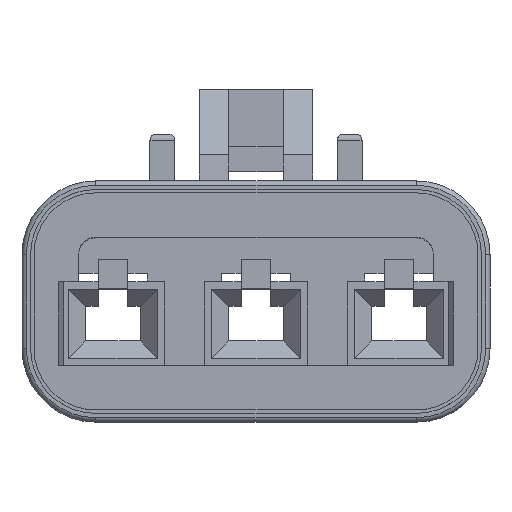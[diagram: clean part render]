
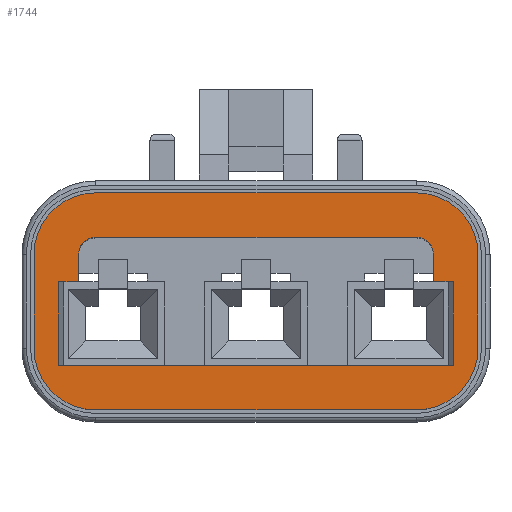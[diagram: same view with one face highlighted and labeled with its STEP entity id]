
A CAD part, top view. The second image highlights one B-rep face of the part: STEP entity #1744.
In plain terms, the highlighted planar face has unit normal (0, 0, 1).
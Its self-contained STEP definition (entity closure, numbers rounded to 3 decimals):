
#148 = VECTOR ( 'NONE', #1796, 1000. ) ;
#175 = AXIS2_PLACEMENT_3D ( 'NONE', #8669, #4275, #6469 ) ;
#259 = VECTOR ( 'NONE', #5581, 1000. ) ;
#351 = LINE ( 'NONE', #9261, #5116 ) ;
#423 = DIRECTION ( 'NONE',  ( 1., 0., 0. ) ) ;
#487 = EDGE_CURVE ( 'NONE', #14204, #9851, #10210, .T. ) ;
#541 = LINE ( 'NONE', #13019, #6979 ) ;
#652 = CARTESIAN_POINT ( 'NONE',  ( 7.2, 2.5, 26. ) ) ;
#702 = VERTEX_POINT ( 'NONE', #5740 ) ;
#755 = CARTESIAN_POINT ( 'NONE',  ( 9., 2.5, 26. ) ) ;
#783 = LINE ( 'NONE', #6271, #148 ) ;
#839 = FACE_BOUND ( 'NONE', #12326, .T. ) ;
#920 = CIRCLE ( 'NONE', #8642, 2.5 ) ;
#995 = DIRECTION ( 'NONE',  ( 0., 0., 1. ) ) ;
#1138 = AXIS2_PLACEMENT_3D ( 'NONE', #12852, #7104, #5040 ) ;
#1155 = ORIENTED_EDGE ( 'NONE', *, *, #10953, .F. ) ;
#1247 = ORIENTED_EDGE ( 'NONE', *, *, #12876, .T. ) ;
#1343 = ORIENTED_EDGE ( 'NONE', *, *, #2974, .T. ) ;
#1395 = DIRECTION ( 'NONE',  ( 0., 1., 0. ) ) ;
#1744 = ADVANCED_FACE ( 'NONE', ( #839, #4198 ), #1860, .T. ) ;
#1796 = DIRECTION ( 'NONE',  ( 1., 0., 0. ) ) ;
#1860 = PLANE ( 'NONE',  #175 ) ;
#2545 = CARTESIAN_POINT ( 'NONE',  ( 8., -2., 26. ) ) ;
#2555 = VECTOR ( 'NONE', #7586, 1000. ) ;
#2592 = LINE ( 'NONE', #5595, #9857 ) ;
#2964 = LINE ( 'NONE', #11877, #12336 ) ;
#2974 = EDGE_CURVE ( 'NONE', #7461, #9075, #12168, .T. ) ;
#3086 = CARTESIAN_POINT ( 'NONE',  ( -9., 2.5, 26. ) ) ;
#3341 = EDGE_CURVE ( 'NONE', #9075, #12950, #11338, .T. ) ;
#3458 = VERTEX_POINT ( 'NONE', #9221 ) ;
#3772 = VECTOR ( 'NONE', #4837, 1000. ) ;
#3777 = DIRECTION ( 'NONE',  ( 0., 0., 1. ) ) ;
#3880 = ORIENTED_EDGE ( 'NONE', *, *, #10201, .T. ) ;
#4079 = CARTESIAN_POINT ( 'NONE',  ( -6.5, 2.5, 26. ) ) ;
#4198 = FACE_OUTER_BOUND ( 'NONE', #9828, .T. ) ;
#4275 = DIRECTION ( 'NONE',  ( 0., 0., 1. ) ) ;
#4295 = ORIENTED_EDGE ( 'NONE', *, *, #10071, .F. ) ;
#4398 = ORIENTED_EDGE ( 'NONE', *, *, #11031, .T. ) ;
#4552 = VERTEX_POINT ( 'NONE', #5878 ) ;
#4837 = DIRECTION ( 'NONE',  ( -1., 0., 0. ) ) ;
#4908 = VERTEX_POINT ( 'NONE', #8935 ) ;
#4914 = DIRECTION ( 'NONE',  ( 0., 1., 0. ) ) ;
#4923 = VERTEX_POINT ( 'NONE', #6957 ) ;
#4965 = CARTESIAN_POINT ( 'NONE',  ( 9., -1.3, 26. ) ) ;
#5040 = DIRECTION ( 'NONE',  ( 1., 0., 0. ) ) ;
#5116 = VECTOR ( 'NONE', #423, 1000. ) ;
#5126 = VERTEX_POINT ( 'NONE', #7763 ) ;
#5185 = VERTEX_POINT ( 'NONE', #2545 ) ;
#5456 = DIRECTION ( 'NONE',  ( -1., 0., 0. ) ) ;
#5581 = DIRECTION ( 'NONE',  ( 0., -1., 0. ) ) ;
#5595 = CARTESIAN_POINT ( 'NONE',  ( 6.5, 5., 26. ) ) ;
#5720 = CARTESIAN_POINT ( 'NONE',  ( -9., 2.5, 26. ) ) ;
#5721 = CARTESIAN_POINT ( 'NONE',  ( 7.2, 1.4, 26. ) ) ;
#5740 = CARTESIAN_POINT ( 'NONE',  ( 6.5, -3.8, 26. ) ) ;
#5805 = VECTOR ( 'NONE', #4914, 1000. ) ;
#5843 = LINE ( 'NONE', #12065, #7610 ) ;
#5878 = CARTESIAN_POINT ( 'NONE',  ( -8., -2., 26. ) ) ;
#5934 = CARTESIAN_POINT ( 'NONE',  ( 6.5, 2.5, 26. ) ) ;
#6152 = ORIENTED_EDGE ( 'NONE', *, *, #9581, .F. ) ;
#6271 = CARTESIAN_POINT ( 'NONE',  ( 6.5, -3.8, 26. ) ) ;
#6279 = VERTEX_POINT ( 'NONE', #8212 ) ;
#6295 = ORIENTED_EDGE ( 'NONE', *, *, #7516, .T. ) ;
#6426 = DIRECTION ( 'NONE',  ( 1., 0., 0. ) ) ;
#6438 = CARTESIAN_POINT ( 'NONE',  ( 6.5, 2.5, 26. ) ) ;
#6469 = DIRECTION ( 'NONE',  ( 1., 0., 0. ) ) ;
#6522 = CIRCLE ( 'NONE', #1138, 2.5 ) ;
#6643 = AXIS2_PLACEMENT_3D ( 'NONE', #6438, #9850, #10873 ) ;
#6698 = DIRECTION ( 'NONE',  ( -1., 0., 0. ) ) ;
#6835 = ORIENTED_EDGE ( 'NONE', *, *, #14141, .T. ) ;
#6957 = CARTESIAN_POINT ( 'NONE',  ( -7.2, 1.4, 26. ) ) ;
#6965 = ORIENTED_EDGE ( 'NONE', *, *, #8897, .F. ) ;
#6979 = VECTOR ( 'NONE', #9442, 1000. ) ;
#7104 = DIRECTION ( 'NONE',  ( 0., 0., 1. ) ) ;
#7365 = CARTESIAN_POINT ( 'NONE',  ( -9., -1.3, 26. ) ) ;
#7435 = ORIENTED_EDGE ( 'NONE', *, *, #10886, .F. ) ;
#7461 = VERTEX_POINT ( 'NONE', #11205 ) ;
#7516 = EDGE_CURVE ( 'NONE', #6279, #7461, #2592, .T. ) ;
#7586 = DIRECTION ( 'NONE',  ( -1., 0., 0. ) ) ;
#7610 = VECTOR ( 'NONE', #14406, 1000. ) ;
#7743 = AXIS2_PLACEMENT_3D ( 'NONE', #10997, #995, #5456 ) ;
#7763 = CARTESIAN_POINT ( 'NONE',  ( 7.2, 1.4, 26. ) ) ;
#7981 = VERTEX_POINT ( 'NONE', #652 ) ;
#8002 = DIRECTION ( 'NONE',  ( 0., -1., 0. ) ) ;
#8136 = LINE ( 'NONE', #5721, #3772 ) ;
#8160 = CARTESIAN_POINT ( 'NONE',  ( 6.5, -1.3, 26. ) ) ;
#8212 = CARTESIAN_POINT ( 'NONE',  ( 6.5, 5., 26. ) ) ;
#8324 = DIRECTION ( 'NONE',  ( 0., 0., 1. ) ) ;
#8443 = EDGE_CURVE ( 'NONE', #5126, #7981, #13817, .T. ) ;
#8575 = LINE ( 'NONE', #755, #5805 ) ;
#8642 = AXIS2_PLACEMENT_3D ( 'NONE', #5934, #8951, #6698 ) ;
#8669 = CARTESIAN_POINT ( 'NONE',  ( -6.5, -1.3, 26. ) ) ;
#8880 = CARTESIAN_POINT ( 'NONE',  ( 9., 2.5, 26. ) ) ;
#8897 = EDGE_CURVE ( 'NONE', #4908, #5126, #8136, .T. ) ;
#8929 = ORIENTED_EDGE ( 'NONE', *, *, #3341, .T. ) ;
#8935 = CARTESIAN_POINT ( 'NONE',  ( 8., 1.4, 26. ) ) ;
#8951 = DIRECTION ( 'NONE',  ( 0., 0., 1. ) ) ;
#9015 = ORIENTED_EDGE ( 'NONE', *, *, #8443, .F. ) ;
#9028 = VERTEX_POINT ( 'NONE', #9574 ) ;
#9075 = VERTEX_POINT ( 'NONE', #3086 ) ;
#9085 = CARTESIAN_POINT ( 'NONE',  ( -7.2, 2.5, 26. ) ) ;
#9087 = ORIENTED_EDGE ( 'NONE', *, *, #487, .F. ) ;
#9192 = CIRCLE ( 'NONE', #6643, 0.7 ) ;
#9221 = CARTESIAN_POINT ( 'NONE',  ( 6.5, 3.2, 26. ) ) ;
#9261 = CARTESIAN_POINT ( 'NONE',  ( -6.5, -2., 26. ) ) ;
#9431 = VERTEX_POINT ( 'NONE', #4965 ) ;
#9442 = DIRECTION ( 'NONE',  ( 0., 1., 0. ) ) ;
#9484 = ORIENTED_EDGE ( 'NONE', *, *, #10559, .T. ) ;
#9574 = CARTESIAN_POINT ( 'NONE',  ( -8., 1.4, 26. ) ) ;
#9581 = EDGE_CURVE ( 'NONE', #7981, #3458, #9192, .T. ) ;
#9828 = EDGE_LOOP ( 'NONE', ( #9484, #6835, #1247, #3880, #4398, #6295, #1343, #8929 ) ) ;
#9850 = DIRECTION ( 'NONE',  ( 0., 0., 1. ) ) ;
#9851 = VERTEX_POINT ( 'NONE', #12078 ) ;
#9857 = VECTOR ( 'NONE', #12302, 1000. ) ;
#9895 = VERTEX_POINT ( 'NONE', #8880 ) ;
#10071 = EDGE_CURVE ( 'NONE', #9851, #4923, #10388, .T. ) ;
#10126 = EDGE_CURVE ( 'NONE', #5185, #4908, #541, .T. ) ;
#10178 = ORIENTED_EDGE ( 'NONE', *, *, #13498, .F. ) ;
#10201 = EDGE_CURVE ( 'NONE', #9431, #9895, #8575, .T. ) ;
#10208 = CIRCLE ( 'NONE', #10451, 2.5 ) ;
#10210 = CIRCLE ( 'NONE', #11394, 0.7 ) ;
#10299 = CARTESIAN_POINT ( 'NONE',  ( -6.5, -3.8, 26. ) ) ;
#10388 = LINE ( 'NONE', #9085, #12324 ) ;
#10451 = AXIS2_PLACEMENT_3D ( 'NONE', #8160, #3777, #12598 ) ;
#10463 = VERTEX_POINT ( 'NONE', #10299 ) ;
#10559 = EDGE_CURVE ( 'NONE', #12950, #10463, #6522, .T. ) ;
#10697 = CARTESIAN_POINT ( 'NONE',  ( 6.5, 3.2, 26. ) ) ;
#10850 = DIRECTION ( 'NONE',  ( -1., 0., 0. ) ) ;
#10855 = CARTESIAN_POINT ( 'NONE',  ( -6.5, 3.2, 26. ) ) ;
#10873 = DIRECTION ( 'NONE',  ( 1., 0., 0. ) ) ;
#10886 = EDGE_CURVE ( 'NONE', #4923, #9028, #2964, .T. ) ;
#10911 = LINE ( 'NONE', #10697, #2555 ) ;
#10953 = EDGE_CURVE ( 'NONE', #3458, #14204, #10911, .T. ) ;
#10969 = VECTOR ( 'NONE', #1395, 1000. ) ;
#10997 = CARTESIAN_POINT ( 'NONE',  ( -6.5, 2.5, 26. ) ) ;
#11031 = EDGE_CURVE ( 'NONE', #9895, #6279, #920, .T. ) ;
#11205 = CARTESIAN_POINT ( 'NONE',  ( -6.5, 5., 26. ) ) ;
#11211 = EDGE_CURVE ( 'NONE', #4552, #5185, #351, .T. ) ;
#11338 = LINE ( 'NONE', #5720, #259 ) ;
#11394 = AXIS2_PLACEMENT_3D ( 'NONE', #4079, #8324, #6426 ) ;
#11647 = ORIENTED_EDGE ( 'NONE', *, *, #11211, .F. ) ;
#11877 = CARTESIAN_POINT ( 'NONE',  ( -7.2, 1.4, 26. ) ) ;
#12065 = CARTESIAN_POINT ( 'NONE',  ( -8., -2., 26. ) ) ;
#12078 = CARTESIAN_POINT ( 'NONE',  ( -7.2, 2.5, 26. ) ) ;
#12168 = CIRCLE ( 'NONE', #7743, 2.5 ) ;
#12302 = DIRECTION ( 'NONE',  ( -1., 0., 0. ) ) ;
#12324 = VECTOR ( 'NONE', #8002, 1000. ) ;
#12326 = EDGE_LOOP ( 'NONE', ( #11647, #10178, #7435, #4295, #9087, #1155, #6152, #9015, #6965, #13838 ) ) ;
#12336 = VECTOR ( 'NONE', #10850, 1000. ) ;
#12598 = DIRECTION ( 'NONE',  ( 1., 0., 0. ) ) ;
#12643 = CARTESIAN_POINT ( 'NONE',  ( 7.2, -1.3, 26. ) ) ;
#12852 = CARTESIAN_POINT ( 'NONE',  ( -6.5, -1.3, 26. ) ) ;
#12876 = EDGE_CURVE ( 'NONE', #702, #9431, #10208, .T. ) ;
#12950 = VERTEX_POINT ( 'NONE', #7365 ) ;
#13019 = CARTESIAN_POINT ( 'NONE',  ( 8., -2., 26. ) ) ;
#13498 = EDGE_CURVE ( 'NONE', #9028, #4552, #5843, .T. ) ;
#13817 = LINE ( 'NONE', #12643, #10969 ) ;
#13838 = ORIENTED_EDGE ( 'NONE', *, *, #10126, .F. ) ;
#14141 = EDGE_CURVE ( 'NONE', #10463, #702, #783, .T. ) ;
#14204 = VERTEX_POINT ( 'NONE', #10855 ) ;
#14406 = DIRECTION ( 'NONE',  ( 0., -1., 0. ) ) ;
